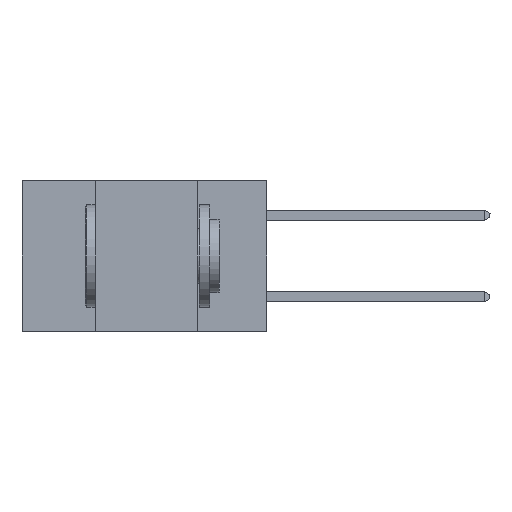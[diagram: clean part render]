
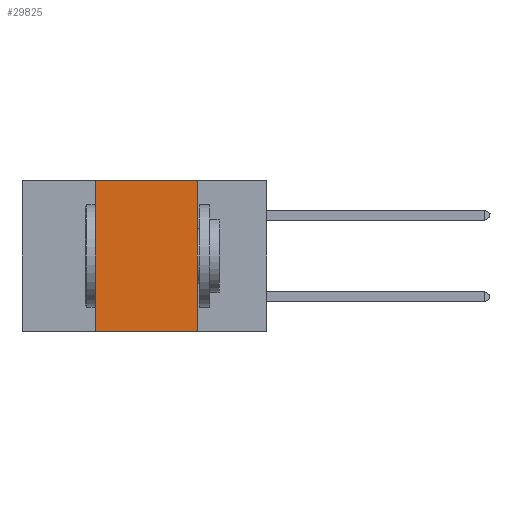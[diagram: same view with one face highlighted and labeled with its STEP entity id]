
A CAD part, left-side view. The second image highlights one B-rep face of the part: STEP entity #29825.
In plain terms, the highlighted planar face has unit normal (-1, 0, 0).
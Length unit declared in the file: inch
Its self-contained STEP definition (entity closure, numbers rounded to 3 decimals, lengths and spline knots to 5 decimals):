
#364 = CARTESIAN_POINT ( 'NONE',  ( 0., 0.6, 0. ) ) ;
#1331 = EDGE_CURVE ( 'NONE', #27677, #18754, #11684, .T. ) ;
#3074 = EDGE_CURVE ( 'NONE', #10872, #24653, #24394, .T. ) ;
#3348 = VECTOR ( 'NONE', #9058, 39.37008 ) ;
#5282 = EDGE_CURVE ( 'NONE', #10872, #18754, #9286, .T. ) ;
#5470 = DIRECTION ( 'NONE',  ( 0., 0., -1. ) ) ;
#7312 = ORIENTED_EDGE ( 'NONE', *, *, #5282, .T. ) ;
#8846 = VECTOR ( 'NONE', #9896, 39.37008 ) ;
#9053 = DIRECTION ( 'NONE',  ( 1., 0., 0. ) ) ;
#9058 = DIRECTION ( 'NONE',  ( 0., 0., -1. ) ) ;
#9286 = LINE ( 'NONE', #26593, #8846 ) ;
#9433 = FACE_OUTER_BOUND ( 'NONE', #18009, .T. ) ;
#9896 = DIRECTION ( 'NONE',  ( 0., -1., 0. ) ) ;
#10872 = VERTEX_POINT ( 'NONE', #27579 ) ;
#11364 = CARTESIAN_POINT ( 'NONE',  ( 0., 0.42, 0. ) ) ;
#11684 = LINE ( 'NONE', #26830, #3348 ) ;
#13206 = VECTOR ( 'NONE', #22006, 39.37008 ) ;
#14193 = PLANE ( 'NONE',  #29116 ) ;
#16809 = ORIENTED_EDGE ( 'NONE', *, *, #1331, .F. ) ;
#18009 = EDGE_LOOP ( 'NONE', ( #16809, #18594, #31537, #7312 ) ) ;
#18594 = ORIENTED_EDGE ( 'NONE', *, *, #30796, .F. ) ;
#18754 = VERTEX_POINT ( 'NONE', #19934 ) ;
#19489 = CARTESIAN_POINT ( 'NONE',  ( 0., 0.6, 0. ) ) ;
#19934 = CARTESIAN_POINT ( 'NONE',  ( 0., 0.17, -0.37 ) ) ;
#20992 = CARTESIAN_POINT ( 'NONE',  ( 0., 0.17, 0. ) ) ;
#21384 = VECTOR ( 'NONE', #21895, 39.37008 ) ;
#21895 = DIRECTION ( 'NONE',  ( 0., -1., 0. ) ) ;
#22006 = DIRECTION ( 'NONE',  ( 0., 0., 1. ) ) ;
#24394 = LINE ( 'NONE', #11364, #13206 ) ;
#24653 = VERTEX_POINT ( 'NONE', #34062 ) ;
#26593 = CARTESIAN_POINT ( 'NONE',  ( 0., 0.6, -0.37 ) ) ;
#26830 = CARTESIAN_POINT ( 'NONE',  ( 0., 0.17, 0. ) ) ;
#27579 = CARTESIAN_POINT ( 'NONE',  ( 0., 0.42, -0.37 ) ) ;
#27677 = VERTEX_POINT ( 'NONE', #20992 ) ;
#29116 = AXIS2_PLACEMENT_3D ( 'NONE', #19489, #9053, #5470 ) ;
#29306 = LINE ( 'NONE', #364, #21384 ) ;
#29825 = ADVANCED_FACE ( 'NONE', ( #9433 ), #14193, .F. ) ;
#30796 = EDGE_CURVE ( 'NONE', #24653, #27677, #29306, .T. ) ;
#31537 = ORIENTED_EDGE ( 'NONE', *, *, #3074, .F. ) ;
#34062 = CARTESIAN_POINT ( 'NONE',  ( 0., 0.42, 0. ) ) ;
